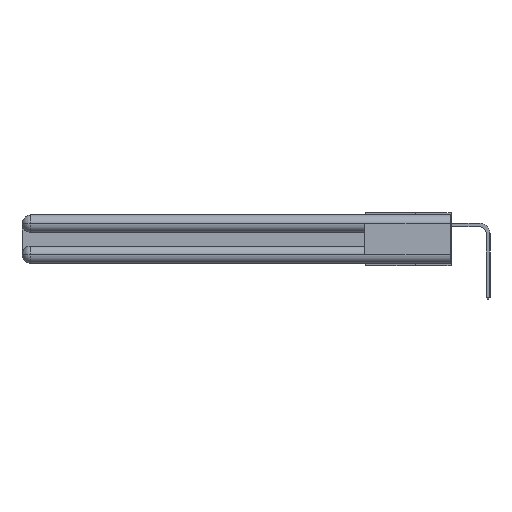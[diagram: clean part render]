
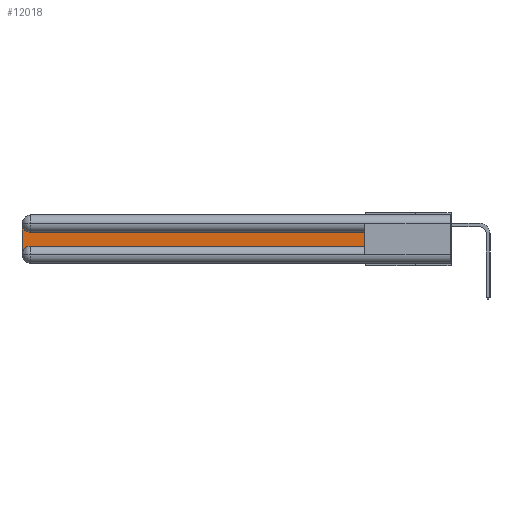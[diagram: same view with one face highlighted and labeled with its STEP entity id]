
A CAD part, left-side view. The second image highlights one B-rep face of the part: STEP entity #12018.
In plain terms, the highlighted planar face has unit normal (-1, 0, 0).
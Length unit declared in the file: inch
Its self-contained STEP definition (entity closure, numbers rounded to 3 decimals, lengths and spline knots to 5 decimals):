
#443 = EDGE_CURVE ( 'NONE', #29743, #3697, #837, .T. ) ;
#837 = LINE ( 'NONE', #27215, #24017 ) ;
#1485 = CARTESIAN_POINT ( 'NONE',  ( 0.075, 0.6, -0.1225 ) ) ;
#2954 = ORIENTED_EDGE ( 'NONE', *, *, #19782, .T. ) ;
#3697 = VERTEX_POINT ( 'NONE', #1485 ) ;
#4150 = EDGE_LOOP ( 'NONE', ( #16678, #2954, #5257, #24350, #21262, #4540 ) ) ;
#4222 = CARTESIAN_POINT ( 'NONE',  ( 0.075, 0.6, -0.1225 ) ) ;
#4540 = ORIENTED_EDGE ( 'NONE', *, *, #443, .T. ) ;
#5257 = ORIENTED_EDGE ( 'NONE', *, *, #31875, .T. ) ;
#5443 = CIRCLE ( 'NONE', #5681, 0.06 ) ;
#5681 = AXIS2_PLACEMENT_3D ( 'NONE', #6850, #9539, #17455 ) ;
#6204 = DIRECTION ( 'NONE',  ( 0., -1., 0. ) ) ;
#6850 = CARTESIAN_POINT ( 'NONE',  ( 0.075, 2.94, -0.2775 ) ) ;
#7462 = CARTESIAN_POINT ( 'NONE',  ( 0.075, 3., -0.1225 ) ) ;
#8421 = VECTOR ( 'NONE', #31592, 39.37008 ) ;
#8795 = DIRECTION ( 'NONE',  ( 0., 0., -1. ) ) ;
#9185 = VECTOR ( 'NONE', #6204, 39.37008 ) ;
#9520 = DIRECTION ( 'NONE',  ( 0., 0., 1. ) ) ;
#9539 = DIRECTION ( 'NONE',  ( 1., 0., 0. ) ) ;
#10181 = DIRECTION ( 'NONE',  ( 1., 0., 0. ) ) ;
#10251 = AXIS2_PLACEMENT_3D ( 'NONE', #7462, #10181, #22139 ) ;
#10551 = FACE_OUTER_BOUND ( 'NONE', #4150, .T. ) ;
#12018 = ADVANCED_FACE ( 'NONE', ( #10551 ), #15147, .F. ) ;
#12540 = CIRCLE ( 'NONE', #32110, 0.06 ) ;
#12992 = EDGE_CURVE ( 'NONE', #29594, #22146, #5443, .T. ) ;
#13085 = LINE ( 'NONE', #4222, #8421 ) ;
#13677 = CARTESIAN_POINT ( 'NONE',  ( 0.075, 2.94, -0.0625 ) ) ;
#14083 = CARTESIAN_POINT ( 'NONE',  ( 0.075, 0.6, -0.2175 ) ) ;
#14103 = CARTESIAN_POINT ( 'NONE',  ( 0.075, 3., -0.0625 ) ) ;
#15147 = PLANE ( 'NONE',  #10251 ) ;
#16358 = CARTESIAN_POINT ( 'NONE',  ( 0.075, 3., -0.2775 ) ) ;
#16404 = DIRECTION ( 'NONE',  ( 1., 0., 0. ) ) ;
#16678 = ORIENTED_EDGE ( 'NONE', *, *, #17685, .T. ) ;
#17455 = DIRECTION ( 'NONE',  ( 0., 0., -1. ) ) ;
#17603 = EDGE_CURVE ( 'NONE', #22146, #29743, #25034, .T. ) ;
#17685 = EDGE_CURVE ( 'NONE', #3697, #30821, #13085, .T. ) ;
#18538 = CARTESIAN_POINT ( 'NONE',  ( 0.075, 3., -0.2175 ) ) ;
#19782 = EDGE_CURVE ( 'NONE', #30821, #29808, #12540, .T. ) ;
#21262 = ORIENTED_EDGE ( 'NONE', *, *, #17603, .T. ) ;
#21753 = LINE ( 'NONE', #18538, #29109 ) ;
#22139 = DIRECTION ( 'NONE',  ( 0., 0., -1. ) ) ;
#22146 = VERTEX_POINT ( 'NONE', #28766 ) ;
#22665 = CARTESIAN_POINT ( 'NONE',  ( 0.075, 0.6, -0.2175 ) ) ;
#24017 = VECTOR ( 'NONE', #9520, 39.37008 ) ;
#24350 = ORIENTED_EDGE ( 'NONE', *, *, #12992, .T. ) ;
#25034 = LINE ( 'NONE', #14083, #9185 ) ;
#26262 = DIRECTION ( 'NONE',  ( 0., 0., -1. ) ) ;
#26790 = CARTESIAN_POINT ( 'NONE',  ( 0.075, 2.94, -0.1225 ) ) ;
#27215 = CARTESIAN_POINT ( 'NONE',  ( 0.075, 0.6, -0.2175 ) ) ;
#28766 = CARTESIAN_POINT ( 'NONE',  ( 0.075, 2.94, -0.2175 ) ) ;
#29109 = VECTOR ( 'NONE', #26262, 39.37008 ) ;
#29594 = VERTEX_POINT ( 'NONE', #16358 ) ;
#29743 = VERTEX_POINT ( 'NONE', #22665 ) ;
#29808 = VERTEX_POINT ( 'NONE', #14103 ) ;
#30821 = VERTEX_POINT ( 'NONE', #26790 ) ;
#31592 = DIRECTION ( 'NONE',  ( 0., 1., 0. ) ) ;
#31875 = EDGE_CURVE ( 'NONE', #29808, #29594, #21753, .T. ) ;
#32110 = AXIS2_PLACEMENT_3D ( 'NONE', #13677, #16404, #8795 ) ;
